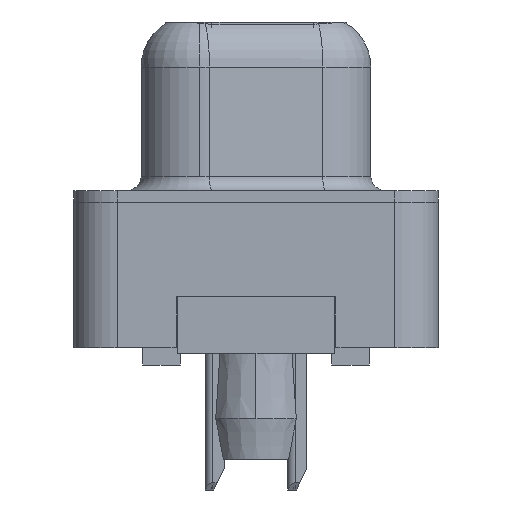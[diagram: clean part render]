
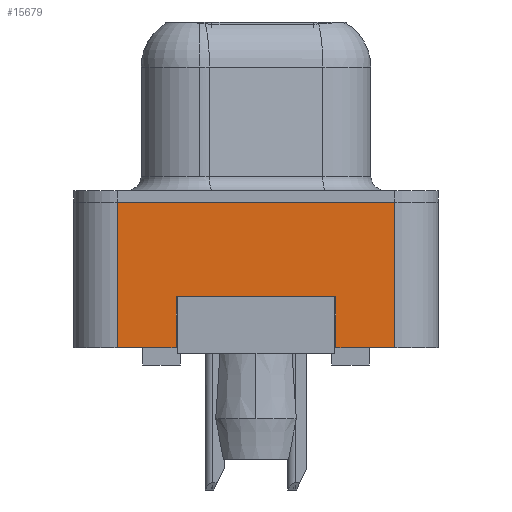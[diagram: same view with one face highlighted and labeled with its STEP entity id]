
A CAD part, left-side view. The second image highlights one B-rep face of the part: STEP entity #15679.
In plain terms, the highlighted planar face has unit normal (-1, 0, 0).
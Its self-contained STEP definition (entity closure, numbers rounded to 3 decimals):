
#130 = CARTESIAN_POINT ( 'NONE',  ( -2.945, -2.75, -3.25 ) ) ;
#149 = EDGE_CURVE ( 'NONE', #6545, #1865, #4332, .T. ) ;
#676 = EDGE_CURVE ( 'NONE', #928, #6573, #16155, .T. ) ;
#928 = VERTEX_POINT ( 'NONE', #130 ) ;
#942 = EDGE_CURVE ( 'NONE', #9680, #2059, #5158, .T. ) ;
#1429 = CARTESIAN_POINT ( 'NONE',  ( -2.945, 2.75, -5. ) ) ;
#1481 = VECTOR ( 'NONE', #1902, 1000. ) ;
#1573 = DIRECTION ( 'NONE',  ( 0., 0., -1. ) ) ;
#1667 = VECTOR ( 'NONE', #6177, 1000. ) ;
#1777 = DIRECTION ( 'NONE',  ( 0., 0., -1. ) ) ;
#1865 = VERTEX_POINT ( 'NONE', #11728 ) ;
#1902 = DIRECTION ( 'NONE',  ( 0., -1., 0. ) ) ;
#2059 = VERTEX_POINT ( 'NONE', #11034 ) ;
#2939 = VECTOR ( 'NONE', #1777, 1000. ) ;
#3017 = ORIENTED_EDGE ( 'NONE', *, *, #4271, .F. ) ;
#3101 = VECTOR ( 'NONE', #1573, 1000. ) ;
#4041 = DIRECTION ( 'NONE',  ( -1., 0., 0. ) ) ;
#4212 = CARTESIAN_POINT ( 'NONE',  ( -2.945, 2.75, -3.25 ) ) ;
#4213 = CARTESIAN_POINT ( 'NONE',  ( -2.945, -4.775, -5. ) ) ;
#4271 = EDGE_CURVE ( 'NONE', #10789, #6545, #5956, .T. ) ;
#4332 = LINE ( 'NONE', #16512, #1481 ) ;
#4574 = CARTESIAN_POINT ( 'NONE',  ( -2.945, 4.775, -5. ) ) ;
#5158 = LINE ( 'NONE', #6636, #15824 ) ;
#5320 = ORIENTED_EDGE ( 'NONE', *, *, #149, .F. ) ;
#5419 = DIRECTION ( 'NONE',  ( 0., -1., 0. ) ) ;
#5860 = DIRECTION ( 'NONE',  ( 0., 1., 0. ) ) ;
#5942 = ORIENTED_EDGE ( 'NONE', *, *, #8686, .T. ) ;
#5956 = LINE ( 'NONE', #4574, #16169 ) ;
#6177 = DIRECTION ( 'NONE',  ( 0., 0., 1. ) ) ;
#6261 = LINE ( 'NONE', #8648, #14493 ) ;
#6431 = CARTESIAN_POINT ( 'NONE',  ( -2.945, -4.775, -5. ) ) ;
#6436 = ORIENTED_EDGE ( 'NONE', *, *, #7390, .T. ) ;
#6545 = VERTEX_POINT ( 'NONE', #9330 ) ;
#6573 = VERTEX_POINT ( 'NONE', #9416 ) ;
#6636 = CARTESIAN_POINT ( 'NONE',  ( -2.945, -4.775, -5. ) ) ;
#6739 = PLANE ( 'NONE',  #11001 ) ;
#6822 = EDGE_CURVE ( 'NONE', #2059, #1865, #13053, .T. ) ;
#6945 = CARTESIAN_POINT ( 'NONE',  ( -2.945, -2.75, -3.25 ) ) ;
#7390 = EDGE_CURVE ( 'NONE', #10789, #13750, #6261, .T. ) ;
#7672 = CARTESIAN_POINT ( 'NONE',  ( -2.945, 4.775, -5. ) ) ;
#8048 = FACE_OUTER_BOUND ( 'NONE', #12872, .T. ) ;
#8648 = CARTESIAN_POINT ( 'NONE',  ( -2.945, -4.775, -5. ) ) ;
#8686 = EDGE_CURVE ( 'NONE', #928, #9680, #12192, .T. ) ;
#9249 = VECTOR ( 'NONE', #5860, 1000. ) ;
#9330 = CARTESIAN_POINT ( 'NONE',  ( -2.945, 4.775, 0. ) ) ;
#9416 = CARTESIAN_POINT ( 'NONE',  ( -2.945, 2.75, -3.25 ) ) ;
#9680 = VERTEX_POINT ( 'NONE', #15088 ) ;
#10021 = ORIENTED_EDGE ( 'NONE', *, *, #676, .F. ) ;
#10789 = VERTEX_POINT ( 'NONE', #7672 ) ;
#10895 = ORIENTED_EDGE ( 'NONE', *, *, #942, .T. ) ;
#11001 = AXIS2_PLACEMENT_3D ( 'NONE', #4213, #4041, #14674 ) ;
#11022 = DIRECTION ( 'NONE',  ( 0., 0., 1. ) ) ;
#11034 = CARTESIAN_POINT ( 'NONE',  ( -2.945, -4.775, -5. ) ) ;
#11728 = CARTESIAN_POINT ( 'NONE',  ( -2.945, -4.775, 0. ) ) ;
#12192 = LINE ( 'NONE', #6945, #3101 ) ;
#12578 = DIRECTION ( 'NONE',  ( 0., -1., 0. ) ) ;
#12872 = EDGE_LOOP ( 'NONE', ( #5942, #10895, #14190, #5320, #3017, #6436, #15367, #10021 ) ) ;
#13053 = LINE ( 'NONE', #6431, #1667 ) ;
#13683 = CARTESIAN_POINT ( 'NONE',  ( -2.945, 2.75, -3.25 ) ) ;
#13750 = VERTEX_POINT ( 'NONE', #1429 ) ;
#13769 = LINE ( 'NONE', #13683, #2939 ) ;
#14190 = ORIENTED_EDGE ( 'NONE', *, *, #6822, .T. ) ;
#14493 = VECTOR ( 'NONE', #12578, 1000. ) ;
#14674 = DIRECTION ( 'NONE',  ( 0., 0., 1. ) ) ;
#15088 = CARTESIAN_POINT ( 'NONE',  ( -2.945, -2.75, -5. ) ) ;
#15367 = ORIENTED_EDGE ( 'NONE', *, *, #15462, .F. ) ;
#15462 = EDGE_CURVE ( 'NONE', #6573, #13750, #13769, .T. ) ;
#15679 = ADVANCED_FACE ( 'NONE', ( #8048 ), #6739, .T. ) ;
#15824 = VECTOR ( 'NONE', #5419, 1000. ) ;
#16155 = LINE ( 'NONE', #4212, #9249 ) ;
#16169 = VECTOR ( 'NONE', #11022, 1000. ) ;
#16512 = CARTESIAN_POINT ( 'NONE',  ( -2.945, -4.775, 0. ) ) ;
